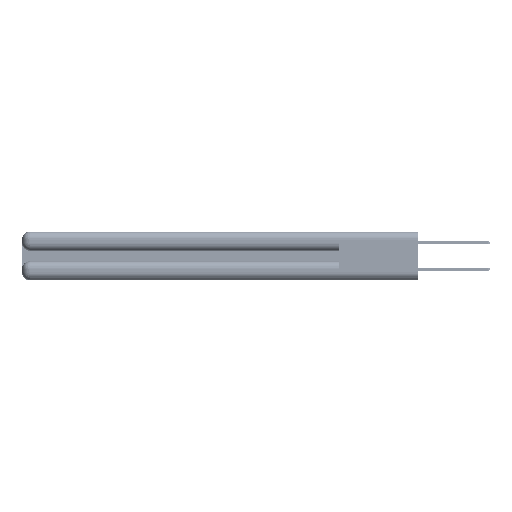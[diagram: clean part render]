
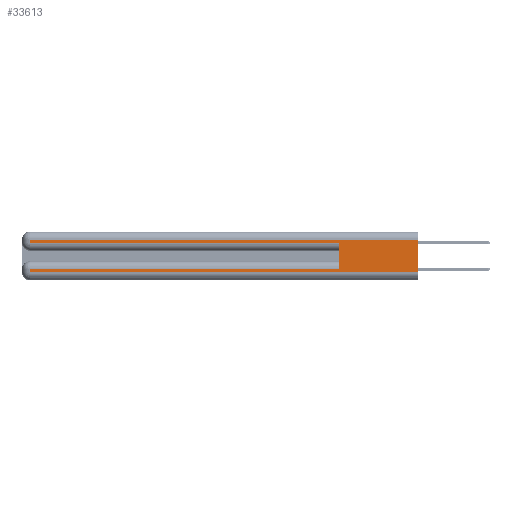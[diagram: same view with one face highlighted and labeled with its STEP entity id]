
A CAD part, left-side view. The second image highlights one B-rep face of the part: STEP entity #33613.
In plain terms, the highlighted planar face has unit normal (-1, 0, 0).
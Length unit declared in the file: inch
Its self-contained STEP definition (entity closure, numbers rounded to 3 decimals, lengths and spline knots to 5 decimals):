
#317 = CARTESIAN_POINT ( 'NONE',  ( 0., 2.94, 0.285 ) ) ;
#326 = CARTESIAN_POINT ( 'NONE',  ( 0., 0.6, 0.145 ) ) ;
#2502 = EDGE_CURVE ( 'NONE', #38802, #11714, #13041, .T. ) ;
#2583 = EDGE_CURVE ( 'NONE', #11714, #16227, #10473, .T. ) ;
#3046 = PLANE ( 'NONE',  #12398 ) ;
#3632 = DIRECTION ( 'NONE',  ( 0., 0., -1. ) ) ;
#4268 = ORIENTED_EDGE ( 'NONE', *, *, #2583, .T. ) ;
#4622 = EDGE_CURVE ( 'NONE', #7880, #13988, #50148, .T. ) ;
#4782 = ORIENTED_EDGE ( 'NONE', *, *, #22050, .T. ) ;
#4956 = ORIENTED_EDGE ( 'NONE', *, *, #2502, .T. ) ;
#5850 = VECTOR ( 'NONE', #33768, 39.37008 ) ;
#7880 = VERTEX_POINT ( 'NONE', #317 ) ;
#8733 = VECTOR ( 'NONE', #3632, 39.37008 ) ;
#9190 = ORIENTED_EDGE ( 'NONE', *, *, #9316, .T. ) ;
#9288 = DIRECTION ( 'NONE',  ( 0., -1., 0. ) ) ;
#9316 = EDGE_CURVE ( 'NONE', #31396, #10735, #35588, .T. ) ;
#9981 = CARTESIAN_POINT ( 'NONE',  ( 0., 2.94, 0.085 ) ) ;
#10473 = LINE ( 'NONE', #15960, #51567 ) ;
#10735 = VERTEX_POINT ( 'NONE', #36440 ) ;
#10844 = CARTESIAN_POINT ( 'NONE',  ( 0., 2.94, 0.37 ) ) ;
#10928 = EDGE_CURVE ( 'NONE', #16227, #28015, #27731, .T. ) ;
#11714 = VERTEX_POINT ( 'NONE', #9981 ) ;
#12398 = AXIS2_PLACEMENT_3D ( 'NONE', #48243, #52375, #27833 ) ;
#13041 = LINE ( 'NONE', #44351, #36144 ) ;
#13194 = ORIENTED_EDGE ( 'NONE', *, *, #20634, .F. ) ;
#13988 = VERTEX_POINT ( 'NONE', #35964 ) ;
#14960 = DIRECTION ( 'NONE',  ( 0., 0., -1. ) ) ;
#15960 = CARTESIAN_POINT ( 'NONE',  ( 0., 2.94, 0.37 ) ) ;
#16227 = VERTEX_POINT ( 'NONE', #17263 ) ;
#17263 = CARTESIAN_POINT ( 'NONE',  ( 0., 2.94, 0.06 ) ) ;
#18660 = VECTOR ( 'NONE', #9288, 39.37008 ) ;
#19640 = LINE ( 'NONE', #44559, #8733 ) ;
#19750 = DIRECTION ( 'NONE',  ( 0., 1., 0. ) ) ;
#20634 = EDGE_CURVE ( 'NONE', #31396, #28015, #19640, .T. ) ;
#22050 = EDGE_CURVE ( 'NONE', #10735, #7880, #45889, .T. ) ;
#27457 = DIRECTION ( 'NONE',  ( 0., 1., 0. ) ) ;
#27731 = LINE ( 'NONE', #29669, #5850 ) ;
#27833 = DIRECTION ( 'NONE',  ( 0., 0., -1. ) ) ;
#28015 = VERTEX_POINT ( 'NONE', #49020 ) ;
#29669 = CARTESIAN_POINT ( 'NONE',  ( 0., 0., 0.06 ) ) ;
#30011 = ORIENTED_EDGE ( 'NONE', *, *, #10928, .T. ) ;
#31396 = VERTEX_POINT ( 'NONE', #49845 ) ;
#33613 = ADVANCED_FACE ( 'NONE', ( #37140 ), #3046, .F. ) ;
#33668 = VECTOR ( 'NONE', #14960, 39.37008 ) ;
#33768 = DIRECTION ( 'NONE',  ( 0., -1., 0. ) ) ;
#33871 = CARTESIAN_POINT ( 'NONE',  ( 0., 0., 0.285 ) ) ;
#33968 = VECTOR ( 'NONE', #45327, 39.37008 ) ;
#35588 = LINE ( 'NONE', #47885, #45264 ) ;
#35964 = CARTESIAN_POINT ( 'NONE',  ( 0., 0.6, 0.285 ) ) ;
#36095 = CARTESIAN_POINT ( 'NONE',  ( 0., 0.6, 0.085 ) ) ;
#36144 = VECTOR ( 'NONE', #19750, 39.37008 ) ;
#36440 = CARTESIAN_POINT ( 'NONE',  ( 0., 2.94, 0.31 ) ) ;
#37140 = FACE_OUTER_BOUND ( 'NONE', #40654, .T. ) ;
#38802 = VERTEX_POINT ( 'NONE', #36095 ) ;
#39069 = ORIENTED_EDGE ( 'NONE', *, *, #52725, .F. ) ;
#40654 = EDGE_LOOP ( 'NONE', ( #13194, #9190, #4782, #49788, #39069, #4956, #4268, #30011 ) ) ;
#44351 = CARTESIAN_POINT ( 'NONE',  ( 0., 0., 0.085 ) ) ;
#44559 = CARTESIAN_POINT ( 'NONE',  ( 0., 0., 0.37 ) ) ;
#44889 = LINE ( 'NONE', #326, #33968 ) ;
#45264 = VECTOR ( 'NONE', #27457, 39.37008 ) ;
#45327 = DIRECTION ( 'NONE',  ( 0., 0., 1. ) ) ;
#45889 = LINE ( 'NONE', #10844, #33668 ) ;
#47885 = CARTESIAN_POINT ( 'NONE',  ( 0., 0., 0.31 ) ) ;
#48243 = CARTESIAN_POINT ( 'NONE',  ( 0., 0., 0.37 ) ) ;
#48637 = DIRECTION ( 'NONE',  ( 0., 0., -1. ) ) ;
#49020 = CARTESIAN_POINT ( 'NONE',  ( 0., 0., 0.06 ) ) ;
#49788 = ORIENTED_EDGE ( 'NONE', *, *, #4622, .T. ) ;
#49845 = CARTESIAN_POINT ( 'NONE',  ( 0., 0., 0.31 ) ) ;
#50148 = LINE ( 'NONE', #33871, #18660 ) ;
#51567 = VECTOR ( 'NONE', #48637, 39.37008 ) ;
#52375 = DIRECTION ( 'NONE',  ( 1., 0., 0. ) ) ;
#52725 = EDGE_CURVE ( 'NONE', #38802, #13988, #44889, .T. ) ;
